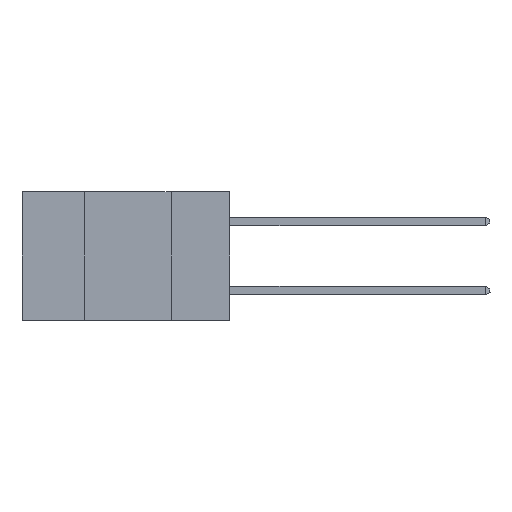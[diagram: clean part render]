
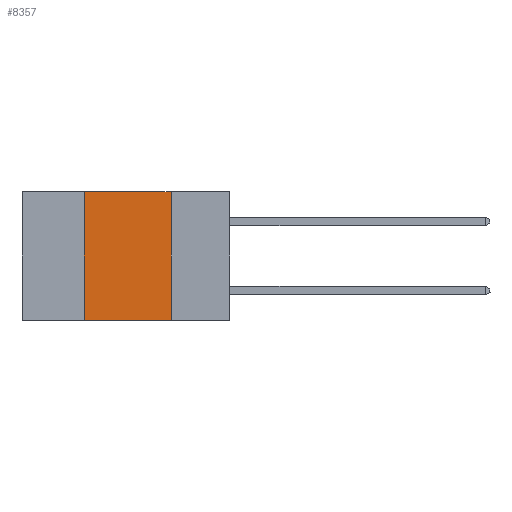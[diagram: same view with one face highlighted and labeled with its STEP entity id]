
A CAD part, left-side view. The second image highlights one B-rep face of the part: STEP entity #8357.
In plain terms, the highlighted planar face has unit normal (-1, 0, 0).
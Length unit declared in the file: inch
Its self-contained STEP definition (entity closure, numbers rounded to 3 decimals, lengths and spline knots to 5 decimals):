
#755 = DIRECTION ( 'NONE',  ( 1., 0., 0. ) ) ;
#1238 = LINE ( 'NONE', #23501, #24569 ) ;
#1973 = DIRECTION ( 'NONE',  ( 0., -1., 0. ) ) ;
#2400 = CARTESIAN_POINT ( 'NONE',  ( 0., 0.17, -0.37 ) ) ;
#4187 = LINE ( 'NONE', #25579, #26517 ) ;
#5629 = CARTESIAN_POINT ( 'NONE',  ( 0., 0.17, 0. ) ) ;
#5678 = EDGE_CURVE ( 'NONE', #15756, #7576, #15049, .T. ) ;
#6192 = DIRECTION ( 'NONE',  ( 0., 0., -1. ) ) ;
#6860 = ORIENTED_EDGE ( 'NONE', *, *, #25912, .T. ) ;
#7576 = VERTEX_POINT ( 'NONE', #5629 ) ;
#7650 = VECTOR ( 'NONE', #1973, 39.37008 ) ;
#8357 = ADVANCED_FACE ( 'NONE', ( #9851 ), #13840, .F. ) ;
#9330 = DIRECTION ( 'NONE',  ( 0., 0., -1. ) ) ;
#9662 = ORIENTED_EDGE ( 'NONE', *, *, #5678, .F. ) ;
#9819 = CARTESIAN_POINT ( 'NONE',  ( 0., 0.42, -0.37 ) ) ;
#9851 = FACE_OUTER_BOUND ( 'NONE', #23435, .T. ) ;
#10766 = ORIENTED_EDGE ( 'NONE', *, *, #21317, .F. ) ;
#10926 = CARTESIAN_POINT ( 'NONE',  ( 0., 0.42, 0. ) ) ;
#11165 = AXIS2_PLACEMENT_3D ( 'NONE', #22683, #755, #9330 ) ;
#13840 = PLANE ( 'NONE',  #11165 ) ;
#14294 = VERTEX_POINT ( 'NONE', #2400 ) ;
#14760 = LINE ( 'NONE', #22875, #18512 ) ;
#15049 = LINE ( 'NONE', #19088, #7650 ) ;
#15756 = VERTEX_POINT ( 'NONE', #10926 ) ;
#18512 = VECTOR ( 'NONE', #18975, 39.37008 ) ;
#18727 = DIRECTION ( 'NONE',  ( 0., -1., 0. ) ) ;
#18975 = DIRECTION ( 'NONE',  ( 0., 0., 1. ) ) ;
#19088 = CARTESIAN_POINT ( 'NONE',  ( 0., 0.6, 0. ) ) ;
#21317 = EDGE_CURVE ( 'NONE', #7576, #14294, #1238, .T. ) ;
#22683 = CARTESIAN_POINT ( 'NONE',  ( 0., 0.6, 0. ) ) ;
#22875 = CARTESIAN_POINT ( 'NONE',  ( 0., 0.42, 0. ) ) ;
#23435 = EDGE_LOOP ( 'NONE', ( #10766, #9662, #25894, #6860 ) ) ;
#23501 = CARTESIAN_POINT ( 'NONE',  ( 0., 0.17, 0. ) ) ;
#23699 = EDGE_CURVE ( 'NONE', #24832, #15756, #14760, .T. ) ;
#24569 = VECTOR ( 'NONE', #6192, 39.37008 ) ;
#24832 = VERTEX_POINT ( 'NONE', #9819 ) ;
#25579 = CARTESIAN_POINT ( 'NONE',  ( 0., 0.6, -0.37 ) ) ;
#25894 = ORIENTED_EDGE ( 'NONE', *, *, #23699, .F. ) ;
#25912 = EDGE_CURVE ( 'NONE', #24832, #14294, #4187, .T. ) ;
#26517 = VECTOR ( 'NONE', #18727, 39.37008 ) ;
